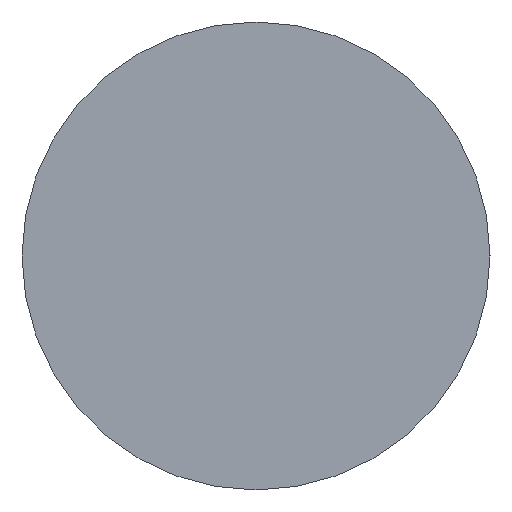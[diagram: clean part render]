
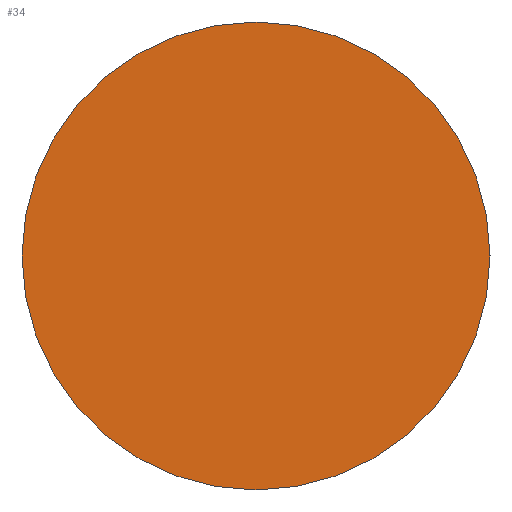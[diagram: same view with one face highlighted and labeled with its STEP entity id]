
A CAD part, left-side view. The second image highlights one B-rep face of the part: STEP entity #34.
In plain terms, the highlighted planar face has unit normal (-1, 0, 0).
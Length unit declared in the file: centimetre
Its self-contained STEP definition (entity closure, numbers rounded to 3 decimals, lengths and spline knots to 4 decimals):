
#15=FACE_OUTER_BOUND($,#18,.T.);
#18=EDGE_LOOP($,(#28));
#22=CIRCLE($,#41,0.4);
#24=VERTEX_POINT($,#59);
#26=EDGE_CURVE($,#24,#24,#22,.T.);
#28=ORIENTED_EDGE($,*,*,#26,.F.);
#32=PLANE($,#40);
#34=ADVANCED_FACE($,(#15),#32,.F.);
#40=AXIS2_PLACEMENT_3D($,#58,#47,#48);
#41=AXIS2_PLACEMENT_3D($,#60,#49,#50);
#47=DIRECTION('center_axis',(1.,0.,0.));
#48=DIRECTION('ref_axis',(0.,0.,-1.));
#49=DIRECTION('center_axis',(1.,0.,0.));
#50=DIRECTION('ref_axis',(0.,0.,-1.));
#58=CARTESIAN_POINT('Origin',(-1.941,4.7829,-2.0721));
#59=CARTESIAN_POINT('',(-1.941,4.7829,-1.6721));
#60=CARTESIAN_POINT('Origin',(-1.941,4.7829,-2.0721));
